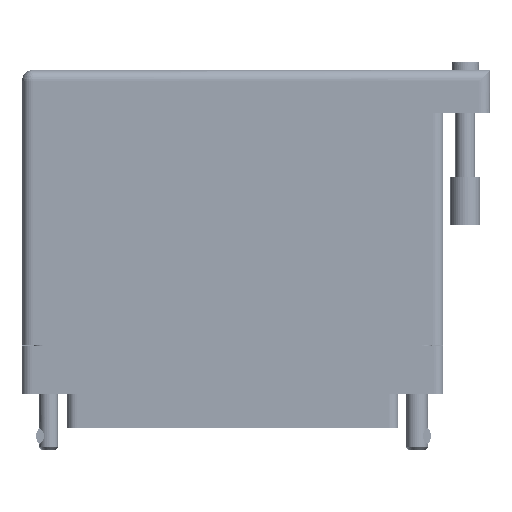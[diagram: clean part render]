
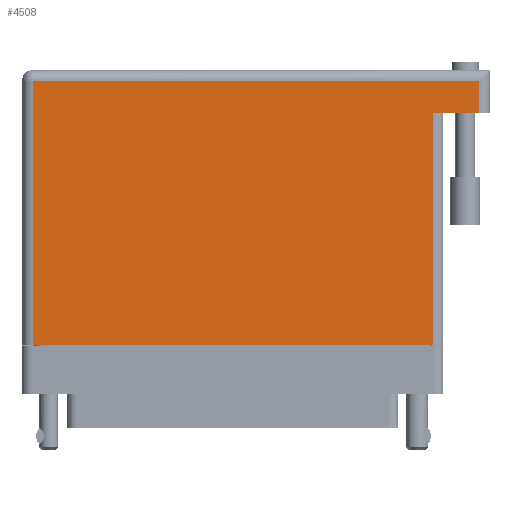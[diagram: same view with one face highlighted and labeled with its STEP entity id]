
A CAD part, front view. The second image highlights one B-rep face of the part: STEP entity #4508.
In plain terms, the highlighted face is planar.
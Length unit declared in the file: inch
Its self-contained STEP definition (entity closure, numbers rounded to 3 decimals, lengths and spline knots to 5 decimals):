
#59 = DIRECTION ( 'NONE',  ( 0., 1., 0. ) ) ;
#444 = VERTEX_POINT ( 'NONE', #57305 ) ;
#912 = VERTEX_POINT ( 'NONE', #79229 ) ;
#4508 = ADVANCED_FACE ( 'NONE', ( #19611 ), #18121, .F. ) ;
#4753 = DIRECTION ( 'NONE',  ( -1., 0., 0. ) ) ;
#7928 = DIRECTION ( 'NONE',  ( 0., -1., 0. ) ) ;
#12370 = VERTEX_POINT ( 'NONE', #68181 ) ;
#13247 = EDGE_CURVE ( 'NONE', #444, #40219, #43275, .T. ) ;
#13818 = CARTESIAN_POINT ( 'NONE',  ( 1.659, 1.395, 0.617 ) ) ;
#14403 = CARTESIAN_POINT ( 'NONE',  ( -1.289, -0.1, 0.617 ) ) ;
#14606 = EDGE_CURVE ( 'NONE', #912, #23814, #33926, .T. ) ;
#15253 = VECTOR ( 'NONE', #4753, 39.37008 ) ;
#15449 = ORIENTED_EDGE ( 'NONE', *, *, #54056, .F. ) ;
#16751 = ORIENTED_EDGE ( 'NONE', *, *, #13247, .T. ) ;
#18121 = PLANE ( 'NONE',  #28274 ) ;
#18987 = VECTOR ( 'NONE', #44040, 39.37008 ) ;
#19611 = FACE_OUTER_BOUND ( 'NONE', #21777, .T. ) ;
#21777 = EDGE_LOOP ( 'NONE', ( #48762, #72817, #15449, #16751, #48520, #32488 ) ) ;
#22331 = VECTOR ( 'NONE', #65523, 39.37008 ) ;
#23814 = VERTEX_POINT ( 'NONE', #42227 ) ;
#23960 = CARTESIAN_POINT ( 'NONE',  ( 1.589, 1.675, 0.617 ) ) ;
#28274 = AXIS2_PLACEMENT_3D ( 'NONE', #82303, #83367, #63634 ) ;
#28872 = EDGE_CURVE ( 'NONE', #40219, #46423, #63744, .T. ) ;
#32488 = ORIENTED_EDGE ( 'NONE', *, *, #40529, .T. ) ;
#33926 = LINE ( 'NONE', #38796, #41029 ) ;
#38796 = CARTESIAN_POINT ( 'NONE',  ( 1.289, 1.395, 0.617 ) ) ;
#39561 = LINE ( 'NONE', #13818, #22331 ) ;
#40219 = VERTEX_POINT ( 'NONE', #42936 ) ;
#40529 = EDGE_CURVE ( 'NONE', #46423, #12370, #52301, .T. ) ;
#41029 = VECTOR ( 'NONE', #59, 39.37008 ) ;
#42227 = CARTESIAN_POINT ( 'NONE',  ( 1.289, 1.395, 0.617 ) ) ;
#42936 = CARTESIAN_POINT ( 'NONE',  ( 1.589, 1.605, 0.617 ) ) ;
#43275 = LINE ( 'NONE', #23960, #18987 ) ;
#44040 = DIRECTION ( 'NONE',  ( 0., 1., 0. ) ) ;
#46423 = VERTEX_POINT ( 'NONE', #70871 ) ;
#47530 = VECTOR ( 'NONE', #83711, 39.37008 ) ;
#48520 = ORIENTED_EDGE ( 'NONE', *, *, #28872, .T. ) ;
#48762 = ORIENTED_EDGE ( 'NONE', *, *, #69209, .T. ) ;
#52301 = LINE ( 'NONE', #14403, #55311 ) ;
#54056 = EDGE_CURVE ( 'NONE', #444, #23814, #39561, .T. ) ;
#54613 = LINE ( 'NONE', #82647, #47530 ) ;
#55311 = VECTOR ( 'NONE', #7928, 39.37008 ) ;
#57305 = CARTESIAN_POINT ( 'NONE',  ( 1.589, 1.395, 0.617 ) ) ;
#63634 = DIRECTION ( 'NONE',  ( -1., 0., 0. ) ) ;
#63744 = LINE ( 'NONE', #75140, #15253 ) ;
#65523 = DIRECTION ( 'NONE',  ( -1., 0., 0. ) ) ;
#68181 = CARTESIAN_POINT ( 'NONE',  ( -1.289, -0.1, 0.617 ) ) ;
#69209 = EDGE_CURVE ( 'NONE', #12370, #912, #54613, .T. ) ;
#70871 = CARTESIAN_POINT ( 'NONE',  ( -1.289, 1.605, 0.617 ) ) ;
#72817 = ORIENTED_EDGE ( 'NONE', *, *, #14606, .T. ) ;
#75140 = CARTESIAN_POINT ( 'NONE',  ( -1.359, 1.605, 0.617 ) ) ;
#79229 = CARTESIAN_POINT ( 'NONE',  ( 1.289, -0.1, 0.617 ) ) ;
#82303 = CARTESIAN_POINT ( 'NONE',  ( -1.359, 1.675, 0.617 ) ) ;
#82647 = CARTESIAN_POINT ( 'NONE',  ( -1.359, -0.1, 0.617 ) ) ;
#83367 = DIRECTION ( 'NONE',  ( 0., 0., -1. ) ) ;
#83711 = DIRECTION ( 'NONE',  ( 1., 0., 0. ) ) ;
